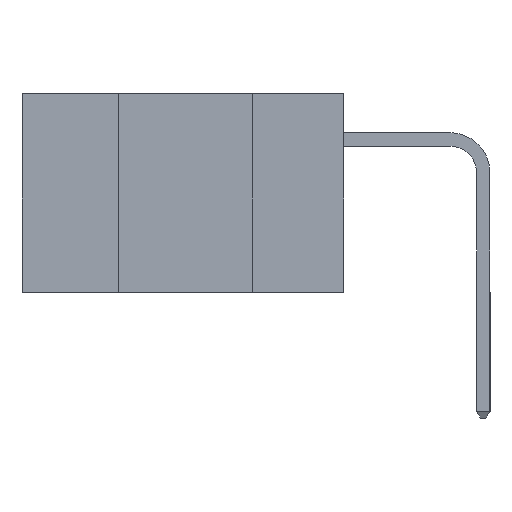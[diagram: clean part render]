
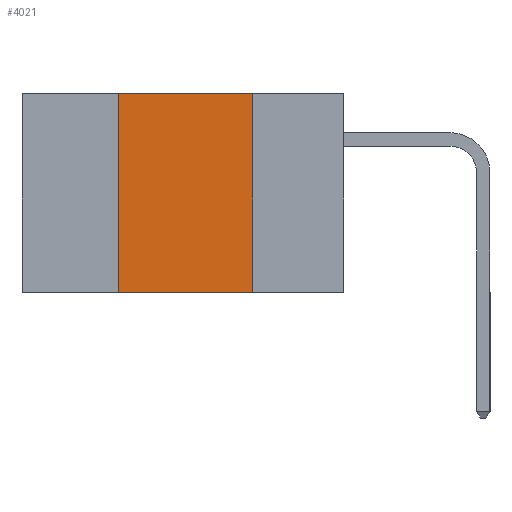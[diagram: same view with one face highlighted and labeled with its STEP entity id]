
A CAD part, left-side view. The second image highlights one B-rep face of the part: STEP entity #4021.
In plain terms, the highlighted planar face has unit normal (-1, 0, 0).
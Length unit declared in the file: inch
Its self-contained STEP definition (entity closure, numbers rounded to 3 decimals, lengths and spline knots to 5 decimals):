
#165 = LINE ( 'NONE', #3733, #3177 ) ;
#768 = DIRECTION ( 'NONE',  ( 0., 0., -1. ) ) ;
#1075 = ORIENTED_EDGE ( 'NONE', *, *, #13518, .F. ) ;
#1287 = ORIENTED_EDGE ( 'NONE', *, *, #9972, .F. ) ;
#1992 = EDGE_LOOP ( 'NONE', ( #1075, #1287, #9559, #8781 ) ) ;
#2822 = VERTEX_POINT ( 'NONE', #7247 ) ;
#3177 = VECTOR ( 'NONE', #15593, 39.37008 ) ;
#3561 = EDGE_CURVE ( 'NONE', #2822, #9774, #11350, .T. ) ;
#3733 = CARTESIAN_POINT ( 'NONE',  ( 0., 0.17, 0. ) ) ;
#3741 = PLANE ( 'NONE',  #8945 ) ;
#4021 = ADVANCED_FACE ( 'NONE', ( #18186 ), #3741, .F. ) ;
#4317 = LINE ( 'NONE', #12252, #7846 ) ;
#4675 = CARTESIAN_POINT ( 'NONE',  ( 0., 0.42, 0. ) ) ;
#4718 = DIRECTION ( 'NONE',  ( 0., 0., 1. ) ) ;
#4744 = DIRECTION ( 'NONE',  ( 0., -1., 0. ) ) ;
#6570 = EDGE_CURVE ( 'NONE', #2822, #9085, #8014, .T. ) ;
#6716 = CARTESIAN_POINT ( 'NONE',  ( 0., 0.42, 0. ) ) ;
#7247 = CARTESIAN_POINT ( 'NONE',  ( 0., 0.42, -0.37 ) ) ;
#7680 = CARTESIAN_POINT ( 'NONE',  ( 0., 0.6, -0.37 ) ) ;
#7846 = VECTOR ( 'NONE', #13709, 39.37008 ) ;
#8014 = LINE ( 'NONE', #4675, #15371 ) ;
#8781 = ORIENTED_EDGE ( 'NONE', *, *, #3561, .T. ) ;
#8945 = AXIS2_PLACEMENT_3D ( 'NONE', #13028, #13008, #768 ) ;
#9085 = VERTEX_POINT ( 'NONE', #6716 ) ;
#9559 = ORIENTED_EDGE ( 'NONE', *, *, #6570, .F. ) ;
#9774 = VERTEX_POINT ( 'NONE', #14687 ) ;
#9972 = EDGE_CURVE ( 'NONE', #9085, #17650, #4317, .T. ) ;
#11350 = LINE ( 'NONE', #7680, #18660 ) ;
#12252 = CARTESIAN_POINT ( 'NONE',  ( 0., 0.6, 0. ) ) ;
#13008 = DIRECTION ( 'NONE',  ( 1., 0., 0. ) ) ;
#13028 = CARTESIAN_POINT ( 'NONE',  ( 0., 0.6, 0. ) ) ;
#13518 = EDGE_CURVE ( 'NONE', #17650, #9774, #165, .T. ) ;
#13709 = DIRECTION ( 'NONE',  ( 0., -1., 0. ) ) ;
#14687 = CARTESIAN_POINT ( 'NONE',  ( 0., 0.17, -0.37 ) ) ;
#15371 = VECTOR ( 'NONE', #4718, 39.37008 ) ;
#15593 = DIRECTION ( 'NONE',  ( 0., 0., -1. ) ) ;
#15914 = CARTESIAN_POINT ( 'NONE',  ( 0., 0.17, 0. ) ) ;
#17650 = VERTEX_POINT ( 'NONE', #15914 ) ;
#18186 = FACE_OUTER_BOUND ( 'NONE', #1992, .T. ) ;
#18660 = VECTOR ( 'NONE', #4744, 39.37008 ) ;
